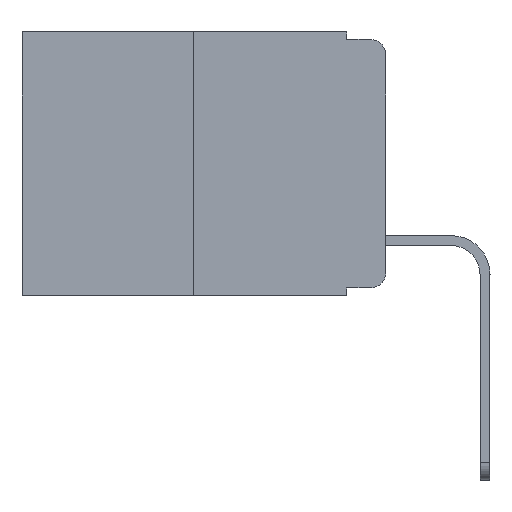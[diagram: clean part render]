
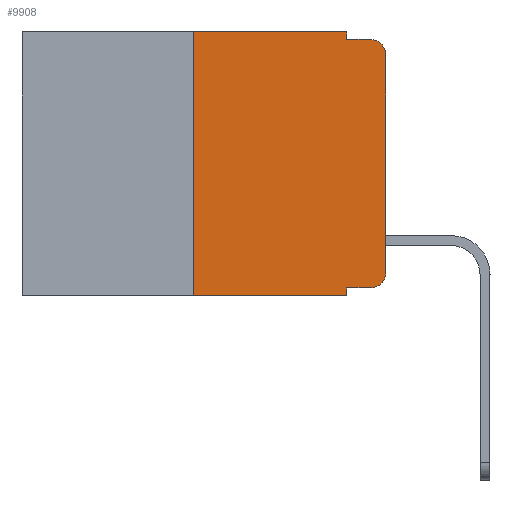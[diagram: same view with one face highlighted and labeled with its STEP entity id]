
A CAD part, left-side view. The second image highlights one B-rep face of the part: STEP entity #9908.
In plain terms, the highlighted planar face has unit normal (-1, 0, 0).
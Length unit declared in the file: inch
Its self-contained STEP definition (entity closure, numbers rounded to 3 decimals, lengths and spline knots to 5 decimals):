
#64 = VERTEX_POINT ( 'NONE', #12902 ) ;
#313 = EDGE_LOOP ( 'NONE', ( #12513, #3293, #13680, #657, #3206, #1107, #7101, #12671, #6304, #1573 ) ) ;
#657 = ORIENTED_EDGE ( 'NONE', *, *, #1714, .F. ) ;
#680 = EDGE_CURVE ( 'NONE', #3533, #14006, #9953, .T. ) ;
#789 = CARTESIAN_POINT ( 'NONE',  ( 0., 0.473, -0.343 ) ) ;
#875 = CARTESIAN_POINT ( 'NONE',  ( 0., 0., -0.03 ) ) ;
#977 = LINE ( 'NONE', #13913, #14138 ) ;
#1028 = DIRECTION ( 'NONE',  ( 0., -1., 0. ) ) ;
#1107 = ORIENTED_EDGE ( 'NONE', *, *, #5125, .F. ) ;
#1313 = EDGE_CURVE ( 'NONE', #64, #11923, #977, .T. ) ;
#1573 = ORIENTED_EDGE ( 'NONE', *, *, #4855, .T. ) ;
#1714 = EDGE_CURVE ( 'NONE', #7337, #3533, #4833, .T. ) ;
#1734 = VECTOR ( 'NONE', #11392, 39.37008 ) ;
#1768 = CARTESIAN_POINT ( 'NONE',  ( 0., 0.02, -0.03 ) ) ;
#1901 = LINE ( 'NONE', #2384, #1734 ) ;
#2384 = CARTESIAN_POINT ( 'NONE',  ( 0., 0., 0. ) ) ;
#2796 = AXIS2_PLACEMENT_3D ( 'NONE', #1768, #7404, #12838 ) ;
#2881 = VECTOR ( 'NONE', #8068, 39.37008 ) ;
#3206 = ORIENTED_EDGE ( 'NONE', *, *, #8748, .F. ) ;
#3293 = ORIENTED_EDGE ( 'NONE', *, *, #11942, .T. ) ;
#3480 = CARTESIAN_POINT ( 'NONE',  ( 0., 0.051, -0.01 ) ) ;
#3533 = VERTEX_POINT ( 'NONE', #7437 ) ;
#3614 = VECTOR ( 'NONE', #9016, 39.37008 ) ;
#3907 = VECTOR ( 'NONE', #5617, 39.37008 ) ;
#4149 = CARTESIAN_POINT ( 'NONE',  ( 0., 0.25, 0. ) ) ;
#4254 = LINE ( 'NONE', #4149, #10940 ) ;
#4440 = EDGE_CURVE ( 'NONE', #9325, #11923, #5837, .T. ) ;
#4668 = CARTESIAN_POINT ( 'NONE',  ( 0., 0.051, -0.333 ) ) ;
#4833 = LINE ( 'NONE', #7843, #3614 ) ;
#4855 = EDGE_CURVE ( 'NONE', #5085, #6904, #11642, .T. ) ;
#4899 = VERTEX_POINT ( 'NONE', #875 ) ;
#5085 = VERTEX_POINT ( 'NONE', #8626 ) ;
#5125 = EDGE_CURVE ( 'NONE', #9325, #9737, #4254, .T. ) ;
#5435 = DIRECTION ( 'NONE',  ( 0., 0., 1. ) ) ;
#5617 = DIRECTION ( 'NONE',  ( 0., -1., 0. ) ) ;
#5772 = AXIS2_PLACEMENT_3D ( 'NONE', #13248, #10965, #11992 ) ;
#5837 = LINE ( 'NONE', #789, #3907 ) ;
#6127 = CARTESIAN_POINT ( 'NONE',  ( 0., 0.051, -0.343 ) ) ;
#6174 = CARTESIAN_POINT ( 'NONE',  ( 0., 0.051, 0. ) ) ;
#6233 = VECTOR ( 'NONE', #1028, 39.37008 ) ;
#6304 = ORIENTED_EDGE ( 'NONE', *, *, #10212, .T. ) ;
#6515 = CARTESIAN_POINT ( 'NONE',  ( 0., 0.02, -0.313 ) ) ;
#6844 = DIRECTION ( 'NONE',  ( 0., -1., 0. ) ) ;
#6904 = VERTEX_POINT ( 'NONE', #10083 ) ;
#7101 = ORIENTED_EDGE ( 'NONE', *, *, #4440, .T. ) ;
#7126 = CARTESIAN_POINT ( 'NONE',  ( 0., 0.25, 0. ) ) ;
#7337 = VERTEX_POINT ( 'NONE', #6174 ) ;
#7404 = DIRECTION ( 'NONE',  ( -1., 0., 0. ) ) ;
#7437 = CARTESIAN_POINT ( 'NONE',  ( 0., 0.051, -0.01 ) ) ;
#7562 = EDGE_CURVE ( 'NONE', #6904, #4899, #1901, .T. ) ;
#7578 = PLANE ( 'NONE',  #5772 ) ;
#7843 = CARTESIAN_POINT ( 'NONE',  ( 0., 0.051, 0. ) ) ;
#8068 = DIRECTION ( 'NONE',  ( 0., -1., 0. ) ) ;
#8214 = VECTOR ( 'NONE', #6844, 39.37008 ) ;
#8335 = FACE_OUTER_BOUND ( 'NONE', #313, .T. ) ;
#8626 = CARTESIAN_POINT ( 'NONE',  ( 0., 0.02, -0.333 ) ) ;
#8748 = EDGE_CURVE ( 'NONE', #9737, #7337, #8892, .T. ) ;
#8892 = LINE ( 'NONE', #12070, #6233 ) ;
#9016 = DIRECTION ( 'NONE',  ( 0., 0., -1. ) ) ;
#9325 = VERTEX_POINT ( 'NONE', #9685 ) ;
#9685 = CARTESIAN_POINT ( 'NONE',  ( 0., 0.25, -0.343 ) ) ;
#9737 = VERTEX_POINT ( 'NONE', #7126 ) ;
#9908 = ADVANCED_FACE ( 'NONE', ( #8335 ), #7578, .F. ) ;
#9953 = LINE ( 'NONE', #3480, #8214 ) ;
#10069 = LINE ( 'NONE', #4668, #2881 ) ;
#10083 = CARTESIAN_POINT ( 'NONE',  ( 0., 0., -0.313 ) ) ;
#10212 = EDGE_CURVE ( 'NONE', #64, #5085, #10069, .T. ) ;
#10401 = AXIS2_PLACEMENT_3D ( 'NONE', #6515, #13290, #14266 ) ;
#10914 = CIRCLE ( 'NONE', #2796, 0.02 ) ;
#10940 = VECTOR ( 'NONE', #5435, 39.37008 ) ;
#10965 = DIRECTION ( 'NONE',  ( 1., 0., 0. ) ) ;
#11392 = DIRECTION ( 'NONE',  ( 0., 0., 1. ) ) ;
#11642 = CIRCLE ( 'NONE', #10401, 0.02 ) ;
#11923 = VERTEX_POINT ( 'NONE', #6127 ) ;
#11942 = EDGE_CURVE ( 'NONE', #4899, #14006, #10914, .T. ) ;
#11992 = DIRECTION ( 'NONE',  ( 0., 0., -1. ) ) ;
#12070 = CARTESIAN_POINT ( 'NONE',  ( 0., 0.473, 0. ) ) ;
#12513 = ORIENTED_EDGE ( 'NONE', *, *, #7562, .T. ) ;
#12671 = ORIENTED_EDGE ( 'NONE', *, *, #1313, .F. ) ;
#12778 = DIRECTION ( 'NONE',  ( 0., 0., -1. ) ) ;
#12838 = DIRECTION ( 'NONE',  ( 0., 0., -1. ) ) ;
#12902 = CARTESIAN_POINT ( 'NONE',  ( 0., 0.051, -0.333 ) ) ;
#13248 = CARTESIAN_POINT ( 'NONE',  ( 0., 0.473, 0. ) ) ;
#13290 = DIRECTION ( 'NONE',  ( -1., 0., 0. ) ) ;
#13680 = ORIENTED_EDGE ( 'NONE', *, *, #680, .F. ) ;
#13913 = CARTESIAN_POINT ( 'NONE',  ( 0., 0.051, 0. ) ) ;
#14006 = VERTEX_POINT ( 'NONE', #14347 ) ;
#14138 = VECTOR ( 'NONE', #12778, 39.37008 ) ;
#14266 = DIRECTION ( 'NONE',  ( 0., 0., -1. ) ) ;
#14347 = CARTESIAN_POINT ( 'NONE',  ( 0., 0.02, -0.01 ) ) ;
